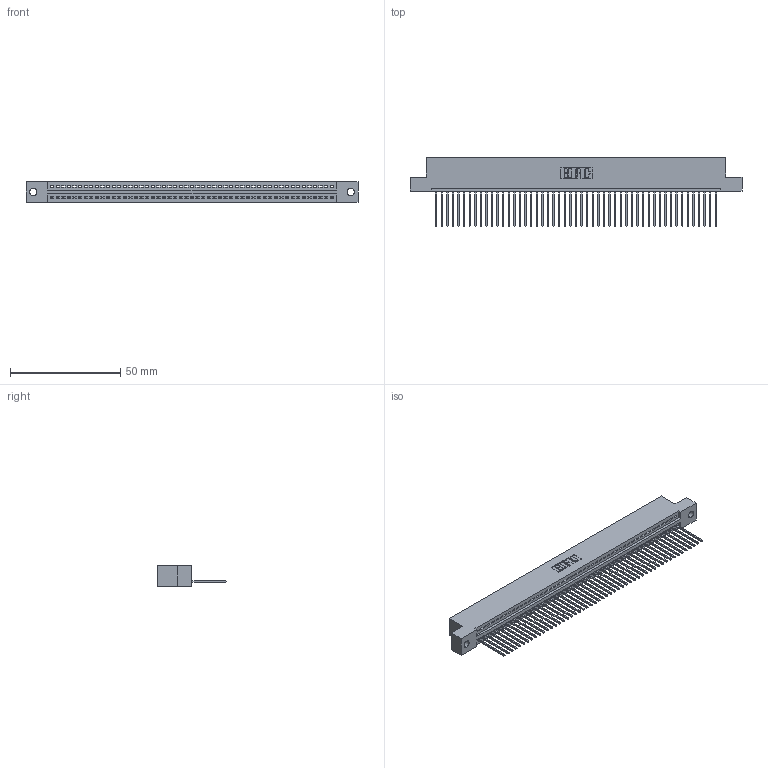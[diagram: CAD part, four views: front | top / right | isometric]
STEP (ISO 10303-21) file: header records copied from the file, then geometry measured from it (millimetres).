
FILE_DESCRIPTION (( 'STEP AP203' ), '1' );
FILE_NAME ('395-051-542-102.STEP', '2018-11-20T18:15:55', ( '' ), ( '' ), 'SwSTEP 2.0', 'SolidWorks 2016', '' );
FILE_SCHEMA (( 'CONFIG_CONTROL_DESIGN' ));
Length unit declared in the file: inch
Products named in the file (3): 395-051-542-102; 345 Part_Flush Mounting Lugs - 0.128 Dia; 345-292-001_345-293-142
Assembly tree (52 placements, depth 2):
  395-051-542-102
    345 Part_Flush Mounting Lugs - 0.128 Dia
    345-292-001_345-293-142  x51
Bounding box: 150.75 x 31.29 x 9.4 mm (x, y, z)
Volume: 14468.8 mm3; surface area: 19796.1 mm2
Topology: 52 solids, 52 shells, 3084 faces, 9317 edges, 6142 vertices
Faces by surface type: plane 2120, cylinder 964
Entity records: 37193 total; most frequent: CARTESIAN_POINT 6449, ORIENTED_EDGE 6434, DIRECTION 5619, EDGE_CURVE 3217, LINE 2881, VECTOR 2881, VERTEX_POINT 2142, AXIS2_PLACEMENT_3D 1369
